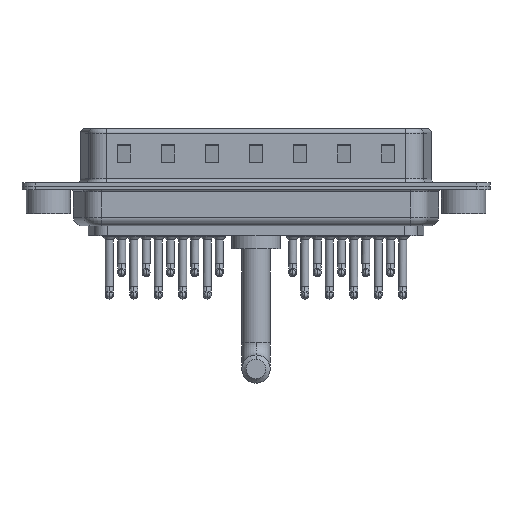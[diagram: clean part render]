
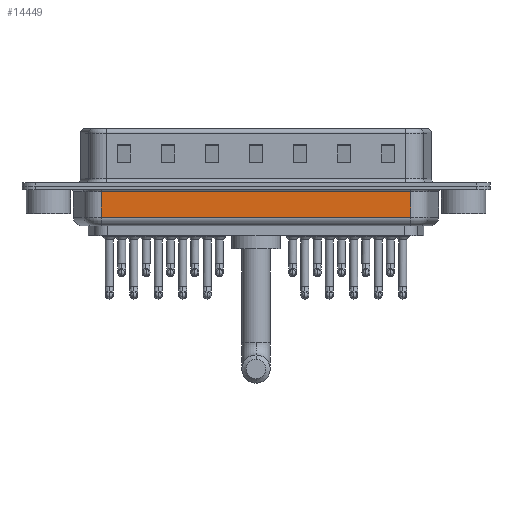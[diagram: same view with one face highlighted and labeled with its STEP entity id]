
A CAD part, front view. The second image highlights one B-rep face of the part: STEP entity #14449.
In plain terms, the highlighted planar face has unit normal (0, -1, 0).
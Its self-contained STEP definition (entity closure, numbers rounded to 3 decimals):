
#1116 = FACE_OUTER_BOUND ( 'NONE', #11342, .T. ) ;
#1291 = EDGE_CURVE ( 'NONE', #7956, #25317, #11223, .T. ) ;
#1429 = ORIENTED_EDGE ( 'NONE', *, *, #17904, .T. ) ;
#1477 = CARTESIAN_POINT ( 'NONE',  ( 41.044, -5.35, -4.5 ) ) ;
#2216 = CARTESIAN_POINT ( 'NONE',  ( 6.006, -5.35, -3.5 ) ) ;
#2372 = VECTOR ( 'NONE', #21302, 1000. ) ;
#3448 = CARTESIAN_POINT ( 'NONE',  ( 6.006, -5.35, -3.5 ) ) ;
#4444 = LINE ( 'NONE', #24481, #7423 ) ;
#7336 = DIRECTION ( 'NONE',  ( -1., 0., 0. ) ) ;
#7423 = VECTOR ( 'NONE', #8648, 1000. ) ;
#7771 = ORIENTED_EDGE ( 'NONE', *, *, #24580, .F. ) ;
#7807 = CARTESIAN_POINT ( 'NONE',  ( 41.044, -5.35, -0.65 ) ) ;
#7956 = VERTEX_POINT ( 'NONE', #18501 ) ;
#8648 = DIRECTION ( 'NONE',  ( 0., 0., 1. ) ) ;
#8959 = LINE ( 'NONE', #3448, #9512 ) ;
#9146 = PLANE ( 'NONE',  #10706 ) ;
#9512 = VECTOR ( 'NONE', #25052, 1000. ) ;
#10706 = AXIS2_PLACEMENT_3D ( 'NONE', #22637, #17151, #12697 ) ;
#11223 = LINE ( 'NONE', #1477, #2372 ) ;
#11342 = EDGE_LOOP ( 'NONE', ( #7771, #1429, #20281, #19282 ) ) ;
#12697 = DIRECTION ( 'NONE',  ( 0., 0., 1. ) ) ;
#14449 = ADVANCED_FACE ( 'NONE', ( #1116 ), #9146, .F. ) ;
#14955 = LINE ( 'NONE', #18904, #14991 ) ;
#14991 = VECTOR ( 'NONE', #7336, 1000. ) ;
#17151 = DIRECTION ( 'NONE',  ( 0., 1., 0. ) ) ;
#17556 = CARTESIAN_POINT ( 'NONE',  ( 6.006, -5.35, -0.65 ) ) ;
#17904 = EDGE_CURVE ( 'NONE', #24550, #7956, #8959, .T. ) ;
#18353 = EDGE_CURVE ( 'NONE', #25317, #24891, #14955, .T. ) ;
#18501 = CARTESIAN_POINT ( 'NONE',  ( 41.044, -5.35, -3.5 ) ) ;
#18904 = CARTESIAN_POINT ( 'NONE',  ( 6.006, -5.35, -0.65 ) ) ;
#19282 = ORIENTED_EDGE ( 'NONE', *, *, #18353, .T. ) ;
#20281 = ORIENTED_EDGE ( 'NONE', *, *, #1291, .T. ) ;
#21302 = DIRECTION ( 'NONE',  ( 0., 0., 1. ) ) ;
#22637 = CARTESIAN_POINT ( 'NONE',  ( 6.006, -5.35, -4.5 ) ) ;
#24481 = CARTESIAN_POINT ( 'NONE',  ( 6.006, -5.35, -4.5 ) ) ;
#24550 = VERTEX_POINT ( 'NONE', #2216 ) ;
#24580 = EDGE_CURVE ( 'NONE', #24550, #24891, #4444, .T. ) ;
#24891 = VERTEX_POINT ( 'NONE', #17556 ) ;
#25052 = DIRECTION ( 'NONE',  ( 1., 0., 0. ) ) ;
#25317 = VERTEX_POINT ( 'NONE', #7807 ) ;
